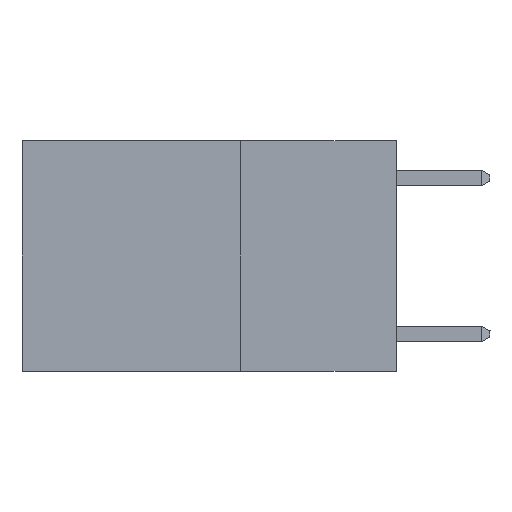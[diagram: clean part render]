
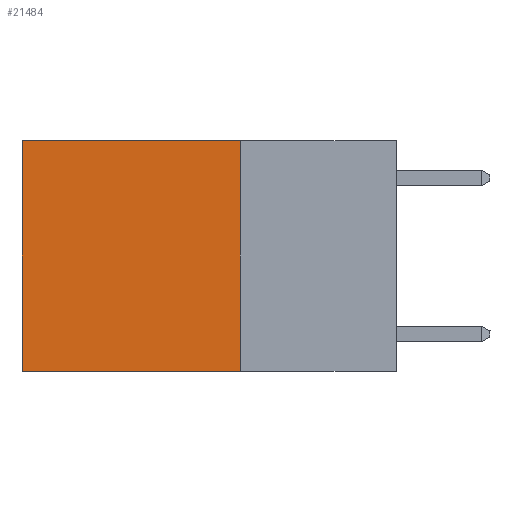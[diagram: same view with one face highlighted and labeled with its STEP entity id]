
A CAD part, left-side view. The second image highlights one B-rep face of the part: STEP entity #21484.
In plain terms, the highlighted planar face has unit normal (-1, 0, 0).
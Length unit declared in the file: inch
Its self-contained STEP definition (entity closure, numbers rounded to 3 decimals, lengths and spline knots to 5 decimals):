
#1792 = CARTESIAN_POINT ( 'NONE',  ( 0.2625, 0.25, 0. ) ) ;
#2168 = CARTESIAN_POINT ( 'NONE',  ( 0.2625, 0.25, -0.37 ) ) ;
#4179 = ORIENTED_EDGE ( 'NONE', *, *, #15283, .T. ) ;
#4598 = DIRECTION ( 'NONE',  ( 0., 1., 0. ) ) ;
#7817 = DIRECTION ( 'NONE',  ( 0., 0., -1. ) ) ;
#8345 = VECTOR ( 'NONE', #28833, 39.37008 ) ;
#8759 = LINE ( 'NONE', #1792, #27365 ) ;
#8887 = PLANE ( 'NONE',  #28727 ) ;
#9003 = VERTEX_POINT ( 'NONE', #27162 ) ;
#9091 = LINE ( 'NONE', #26422, #8345 ) ;
#10611 = ORIENTED_EDGE ( 'NONE', *, *, #16608, .F. ) ;
#11977 = CARTESIAN_POINT ( 'NONE',  ( 0.2625, 0.6, 0. ) ) ;
#12725 = FACE_OUTER_BOUND ( 'NONE', #25286, .T. ) ;
#12827 = VECTOR ( 'NONE', #4598, 39.37008 ) ;
#13796 = DIRECTION ( 'NONE',  ( 0., 0., -1. ) ) ;
#14636 = EDGE_CURVE ( 'NONE', #9003, #22752, #8759, .T. ) ;
#15283 = EDGE_CURVE ( 'NONE', #22752, #17633, #9091, .T. ) ;
#16608 = EDGE_CURVE ( 'NONE', #17973, #17633, #29855, .T. ) ;
#17633 = VERTEX_POINT ( 'NONE', #20324 ) ;
#17973 = VERTEX_POINT ( 'NONE', #23977 ) ;
#18923 = DIRECTION ( 'NONE',  ( 0., 1., 0. ) ) ;
#19838 = VECTOR ( 'NONE', #7817, 39.37008 ) ;
#20324 = CARTESIAN_POINT ( 'NONE',  ( 0.2625, 0.6, -0.37 ) ) ;
#21276 = ORIENTED_EDGE ( 'NONE', *, *, #24762, .F. ) ;
#21484 = ADVANCED_FACE ( 'NONE', ( #12725 ), #8887, .F. ) ;
#22187 = ORIENTED_EDGE ( 'NONE', *, *, #14636, .T. ) ;
#22486 = CARTESIAN_POINT ( 'NONE',  ( 0.2625, 0.25, 0. ) ) ;
#22752 = VERTEX_POINT ( 'NONE', #11977 ) ;
#23977 = CARTESIAN_POINT ( 'NONE',  ( 0.2625, 0.25, -0.37 ) ) ;
#24762 = EDGE_CURVE ( 'NONE', #9003, #17973, #26278, .T. ) ;
#25286 = EDGE_LOOP ( 'NONE', ( #4179, #10611, #21276, #22187 ) ) ;
#25893 = CARTESIAN_POINT ( 'NONE',  ( 0.2625, 0.25, 0. ) ) ;
#26278 = LINE ( 'NONE', #22486, #19838 ) ;
#26422 = CARTESIAN_POINT ( 'NONE',  ( 0.2625, 0.6, 0. ) ) ;
#27162 = CARTESIAN_POINT ( 'NONE',  ( 0.2625, 0.25, 0. ) ) ;
#27365 = VECTOR ( 'NONE', #18923, 39.37008 ) ;
#28318 = DIRECTION ( 'NONE',  ( 1., 0., 0. ) ) ;
#28727 = AXIS2_PLACEMENT_3D ( 'NONE', #25893, #28318, #13796 ) ;
#28833 = DIRECTION ( 'NONE',  ( 0., 0., -1. ) ) ;
#29855 = LINE ( 'NONE', #2168, #12827 ) ;
